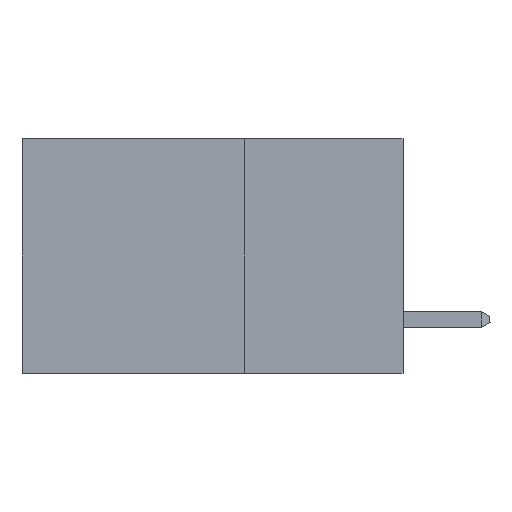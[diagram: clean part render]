
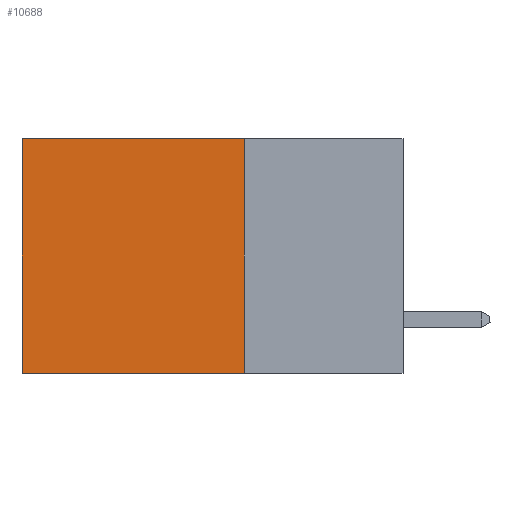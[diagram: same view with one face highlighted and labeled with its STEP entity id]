
A CAD part, left-side view. The second image highlights one B-rep face of the part: STEP entity #10688.
In plain terms, the highlighted planar face has unit normal (-1, 0, 0).
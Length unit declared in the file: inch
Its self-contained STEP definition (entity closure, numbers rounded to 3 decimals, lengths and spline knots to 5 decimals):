
#190 = AXIS2_PLACEMENT_3D ( 'NONE', #15611, #13424, #5102 ) ;
#385 = VERTEX_POINT ( 'NONE', #36121 ) ;
#3128 = VERTEX_POINT ( 'NONE', #31463 ) ;
#3555 = CARTESIAN_POINT ( 'NONE',  ( 0.2875, 0.25, 0. ) ) ;
#4229 = VECTOR ( 'NONE', #23300, 39.37008 ) ;
#4564 = LINE ( 'NONE', #25725, #19506 ) ;
#5102 = DIRECTION ( 'NONE',  ( 0., 0., -1. ) ) ;
#6302 = VERTEX_POINT ( 'NONE', #3555 ) ;
#7817 = CARTESIAN_POINT ( 'NONE',  ( 0.2875, 0.25, 0. ) ) ;
#8510 = EDGE_LOOP ( 'NONE', ( #15724, #24599, #29529, #32773 ) ) ;
#9962 = PLANE ( 'NONE',  #190 ) ;
#10688 = ADVANCED_FACE ( 'NONE', ( #14197 ), #9962, .F. ) ;
#11230 = LINE ( 'NONE', #11953, #4229 ) ;
#11701 = VECTOR ( 'NONE', #29462, 39.37008 ) ;
#11953 = CARTESIAN_POINT ( 'NONE',  ( 0.2875, 0.6, 0. ) ) ;
#12869 = DIRECTION ( 'NONE',  ( 0., 0., -1. ) ) ;
#13424 = DIRECTION ( 'NONE',  ( 1., 0., 0. ) ) ;
#14197 = FACE_OUTER_BOUND ( 'NONE', #8510, .T. ) ;
#15611 = CARTESIAN_POINT ( 'NONE',  ( 0.2875, 0.25, 0. ) ) ;
#15724 = ORIENTED_EDGE ( 'NONE', *, *, #32087, .T. ) ;
#16647 = CARTESIAN_POINT ( 'NONE',  ( 0.2875, 0.25, 0. ) ) ;
#18572 = VECTOR ( 'NONE', #12869, 39.37008 ) ;
#19441 = EDGE_CURVE ( 'NONE', #6302, #19846, #32955, .T. ) ;
#19506 = VECTOR ( 'NONE', #34128, 39.37008 ) ;
#19846 = VERTEX_POINT ( 'NONE', #33112 ) ;
#23300 = DIRECTION ( 'NONE',  ( 0., 0., -1. ) ) ;
#24599 = ORIENTED_EDGE ( 'NONE', *, *, #33165, .F. ) ;
#25725 = CARTESIAN_POINT ( 'NONE',  ( 0.2875, 0.25, -0.37 ) ) ;
#26137 = LINE ( 'NONE', #7817, #18572 ) ;
#29462 = DIRECTION ( 'NONE',  ( 0., 1., 0. ) ) ;
#29529 = ORIENTED_EDGE ( 'NONE', *, *, #34102, .F. ) ;
#31463 = CARTESIAN_POINT ( 'NONE',  ( 0.2875, 0.25, -0.37 ) ) ;
#32087 = EDGE_CURVE ( 'NONE', #19846, #385, #11230, .T. ) ;
#32773 = ORIENTED_EDGE ( 'NONE', *, *, #19441, .T. ) ;
#32955 = LINE ( 'NONE', #16647, #11701 ) ;
#33112 = CARTESIAN_POINT ( 'NONE',  ( 0.2875, 0.6, 0. ) ) ;
#33165 = EDGE_CURVE ( 'NONE', #3128, #385, #4564, .T. ) ;
#34102 = EDGE_CURVE ( 'NONE', #6302, #3128, #26137, .T. ) ;
#34128 = DIRECTION ( 'NONE',  ( 0., 1., 0. ) ) ;
#36121 = CARTESIAN_POINT ( 'NONE',  ( 0.2875, 0.6, -0.37 ) ) ;
